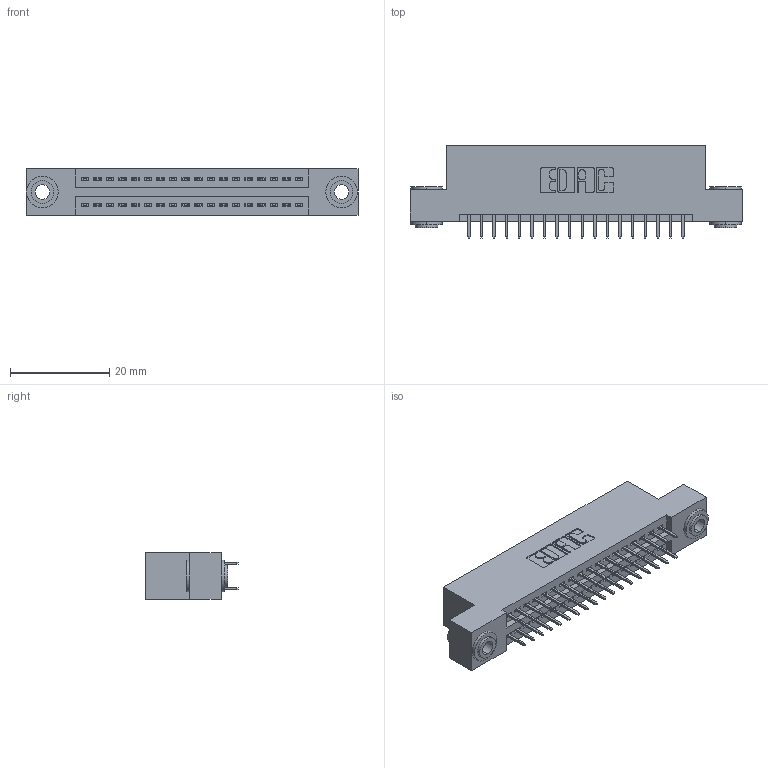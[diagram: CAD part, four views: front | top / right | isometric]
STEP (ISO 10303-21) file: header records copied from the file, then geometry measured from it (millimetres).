
FILE_DESCRIPTION (( 'STEP AP203' ), '1' );
FILE_NAME ('895-036-525-203.STEP', '2020-09-25T23:34:57', ( '' ), ( '' ), 'SwSTEP 2.0', 'SolidWorks 2020', '' );
FILE_SCHEMA (( 'CONFIG_CONTROL_DESIGN' ));
Length unit declared in the file: inch
Products named in the file (4): 895-036-525-203; 345-292-001_345-293-125; 345-250-002_345-250-002-102; 845 Part_Flush Mounting Lugs - 0.156 Dia-TH
Assembly tree (39 placements, depth 2):
  895-036-525-203
    845 Part_Flush Mounting Lugs - 0.156 Dia-TH
    345-292-001_345-293-125  x36
    345-250-002_345-250-002-102  x2
Bounding box: 66.93 x 18.72 x 9.4 mm (x, y, z)
Volume: 6238.9 mm3; surface area: 8783.7 mm2
Topology: 39 solids, 39 shells, 2108 faces, 5925 edges, 3802 vertices
Faces by surface type: plane 1494, cylinder 606, cone 8
Entity records: 18078 total; most frequent: CARTESIAN_POINT 3027, ORIENTED_EDGE 2954, DIRECTION 2731, EDGE_CURVE 1477, VECTOR 1253, LINE 1253, VERTEX_POINT 978, AXIS2_PLACEMENT_3D 739
